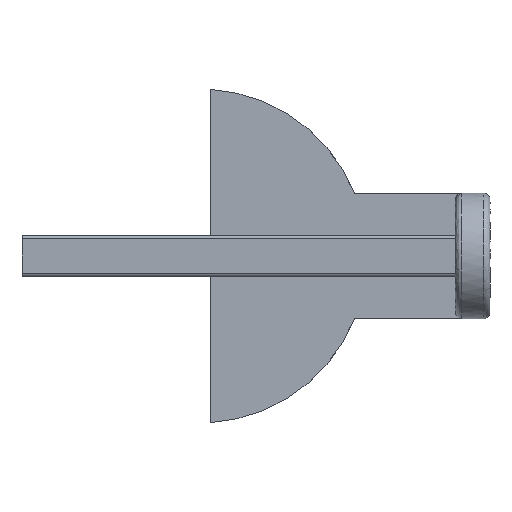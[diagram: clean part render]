
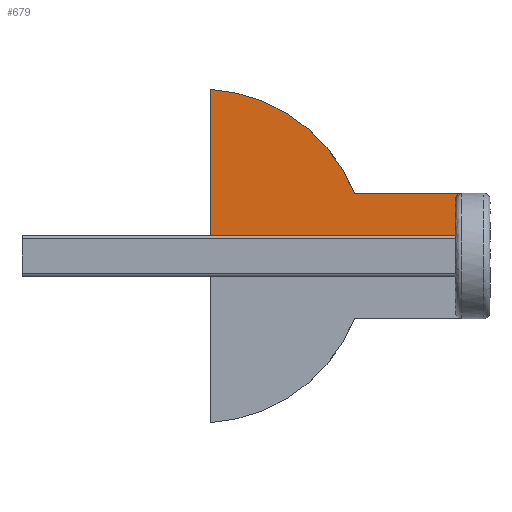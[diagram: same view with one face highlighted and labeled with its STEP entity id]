
A CAD part, left-side view. The second image highlights one B-rep face of the part: STEP entity #679.
In plain terms, the highlighted planar face has unit normal (-1, 0, 0).
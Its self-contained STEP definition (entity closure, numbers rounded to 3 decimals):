
#3 = PLANE ( 'NONE',  #172 ) ;
#27 = EDGE_CURVE ( 'NONE', #907, #207, #811, .T. ) ;
#29 = ORIENTED_EDGE ( 'NONE', *, *, #27, .F. ) ;
#30 = CARTESIAN_POINT ( 'NONE',  ( -207.748, 34.829, 1. ) ) ;
#42 = CARTESIAN_POINT ( 'NONE',  ( -207.748, -6.878, 10.95 ) ) ;
#64 = CARTESIAN_POINT ( 'NONE',  ( -207.748, -6.373, 10.822 ) ) ;
#74 = CARTESIAN_POINT ( 'NONE',  ( -207.748, -5.878, 29.808 ) ) ;
#75 = EDGE_CURVE ( 'NONE', #727, #762, #158, .T. ) ;
#79 = DIRECTION ( 'NONE',  ( 0., 0., -1. ) ) ;
#84 = EDGE_CURVE ( 'NONE', #929, #762, #392, .T. ) ;
#143 = VERTEX_POINT ( 'NONE', #898 ) ;
#145 = CARTESIAN_POINT ( 'NONE',  ( -207.748, -6.878, 10.95 ) ) ;
#149 = LINE ( 'NONE', #74, #236 ) ;
#158 = LINE ( 'NONE', #167, #837 ) ;
#167 = CARTESIAN_POINT ( 'NONE',  ( -207.748, 33.134, 27.537 ) ) ;
#172 = AXIS2_PLACEMENT_3D ( 'NONE', #653, #809, #455 ) ;
#173 = CARTESIAN_POINT ( 'NONE',  ( -207.748, 33.134, 4.25 ) ) ;
#203 = AXIS2_PLACEMENT_3D ( 'NONE', #30, #460, #553 ) ;
#207 = VERTEX_POINT ( 'NONE', #42 ) ;
#213 = CARTESIAN_POINT ( 'NONE',  ( -207.748, 33.134, 27.537 ) ) ;
#236 = VECTOR ( 'NONE', #532, 1000. ) ;
#237 = DIRECTION ( 'NONE',  ( 0., 1., 0. ) ) ;
#240 = CARTESIAN_POINT ( 'NONE',  ( -207.748, -6.746, 10.95 ) ) ;
#259 = EDGE_CURVE ( 'NONE', #143, #929, #149, .T. ) ;
#272 = EDGE_LOOP ( 'NONE', ( #777, #29, #543, #731, #880, #660 ) ) ;
#289 = EDGE_CURVE ( 'NONE', #207, #143, #646, .T. ) ;
#303 = DIRECTION ( 'NONE',  ( 0., -1., 0. ) ) ;
#308 = CARTESIAN_POINT ( 'NONE',  ( -207.748, -6.616, 10.924 ) ) ;
#323 = VECTOR ( 'NONE', #303, 1000. ) ;
#390 = CARTESIAN_POINT ( 'NONE',  ( -207.748, 10.169, 10.95 ) ) ;
#392 = LINE ( 'NONE', #173, #804 ) ;
#455 = DIRECTION ( 'NONE',  ( 0., 0., -1. ) ) ;
#460 = DIRECTION ( 'NONE',  ( 1., 0., 0. ) ) ;
#473 = CARTESIAN_POINT ( 'NONE',  ( -207.748, 4.622, 10.95 ) ) ;
#531 = FACE_OUTER_BOUND ( 'NONE', #272, .T. ) ;
#532 = DIRECTION ( 'NONE',  ( 0., 0., -1. ) ) ;
#543 = ORIENTED_EDGE ( 'NONE', *, *, #848, .F. ) ;
#553 = DIRECTION ( 'NONE',  ( 0., 0., -1. ) ) ;
#596 = CARTESIAN_POINT ( 'NONE',  ( -207.748, -5.878, 10.209 ) ) ;
#646 = B_SPLINE_CURVE_WITH_KNOTS ( 'NONE', 3,
 ( #145, #240, #308, #64, #803, #781, #596, #663 ),
 .UNSPECIFIED., .F., .F.,
 ( 4, 2, 2, 4 ),
 ( 0., 0., 0.001, 0.002 ),
 .UNSPECIFIED. ) ;
#653 = CARTESIAN_POINT ( 'NONE',  ( -207.748, 33.134, 29.808 ) ) ;
#660 = ORIENTED_EDGE ( 'NONE', *, *, #259, .F. ) ;
#663 = CARTESIAN_POINT ( 'NONE',  ( -207.748, -5.878, 9.944 ) ) ;
#679 = ADVANCED_FACE ( 'NONE', ( #531 ), #3, .F. ) ;
#724 = CIRCLE ( 'NONE', #203, 26.591 ) ;
#727 = VERTEX_POINT ( 'NONE', #213 ) ;
#731 = ORIENTED_EDGE ( 'NONE', *, *, #75, .T. ) ;
#757 = CARTESIAN_POINT ( 'NONE',  ( -207.748, -5.878, 4.25 ) ) ;
#762 = VERTEX_POINT ( 'NONE', #790 ) ;
#777 = ORIENTED_EDGE ( 'NONE', *, *, #289, .F. ) ;
#781 = CARTESIAN_POINT ( 'NONE',  ( -207.748, -5.986, 10.469 ) ) ;
#790 = CARTESIAN_POINT ( 'NONE',  ( -207.748, 33.134, 4.25 ) ) ;
#803 = CARTESIAN_POINT ( 'NONE',  ( -207.748, -6.262, 10.747 ) ) ;
#804 = VECTOR ( 'NONE', #237, 1000. ) ;
#809 = DIRECTION ( 'NONE',  ( 1., 0., 0. ) ) ;
#811 = LINE ( 'NONE', #473, #323 ) ;
#837 = VECTOR ( 'NONE', #79, 1000. ) ;
#848 = EDGE_CURVE ( 'NONE', #727, #907, #724, .T. ) ;
#880 = ORIENTED_EDGE ( 'NONE', *, *, #84, .F. ) ;
#898 = CARTESIAN_POINT ( 'NONE',  ( -207.748, -5.878, 9.944 ) ) ;
#907 = VERTEX_POINT ( 'NONE', #390 ) ;
#929 = VERTEX_POINT ( 'NONE', #757 ) ;
